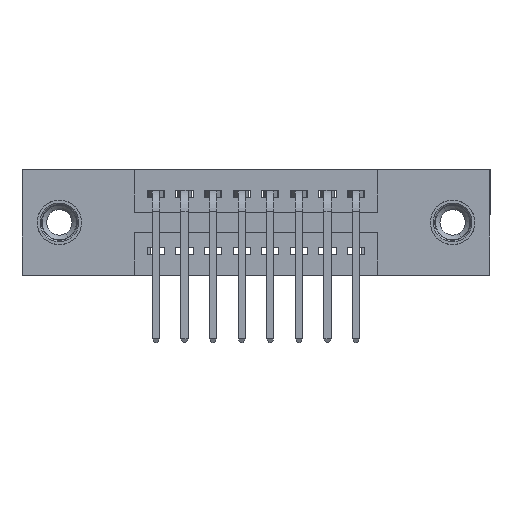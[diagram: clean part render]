
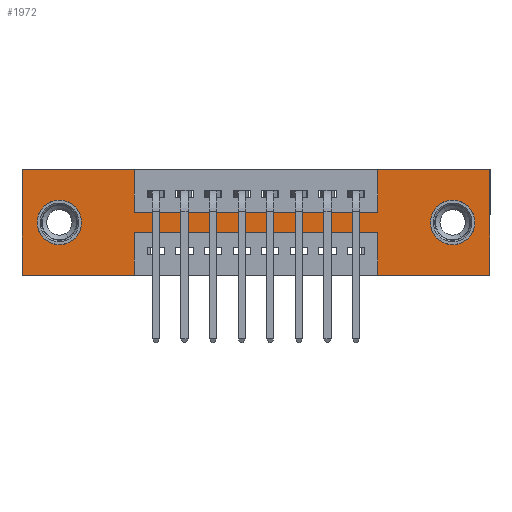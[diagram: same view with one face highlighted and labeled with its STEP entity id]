
A CAD part, front view. The second image highlights one B-rep face of the part: STEP entity #1972.
In plain terms, the highlighted planar face has unit normal (0, -1, 0).
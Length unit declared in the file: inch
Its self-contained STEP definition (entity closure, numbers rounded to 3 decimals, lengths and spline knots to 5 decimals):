
#18 = VECTOR ( 'NONE', #13733, 39.37008 ) ;
#299 = EDGE_LOOP ( 'NONE', ( #1664, #1999 ) ) ;
#496 = DIRECTION ( 'NONE',  ( 0., 1., 0. ) ) ;
#534 = DIRECTION ( 'NONE',  ( -1., 0., 0. ) ) ;
#543 = ORIENTED_EDGE ( 'NONE', *, *, #670, .F. ) ;
#641 = VECTOR ( 'NONE', #14571, 39.37008 ) ;
#670 = EDGE_CURVE ( 'NONE', #12947, #8249, #6791, .T. ) ;
#682 = EDGE_CURVE ( 'NONE', #10014, #4929, #6561, .T. ) ;
#694 = ORIENTED_EDGE ( 'NONE', *, *, #15339, .F. ) ;
#734 = CARTESIAN_POINT ( 'NONE',  ( 0., 0., 0. ) ) ;
#737 = CIRCLE ( 'NONE', #2516, 0.078 ) ;
#743 = LINE ( 'NONE', #13622, #641 ) ;
#760 = VECTOR ( 'NONE', #11612, 39.37008 ) ;
#789 = DIRECTION ( 'NONE',  ( 1., 0., 0. ) ) ;
#1268 = VERTEX_POINT ( 'NONE', #12419 ) ;
#1506 = LINE ( 'NONE', #7781, #1618 ) ;
#1618 = VECTOR ( 'NONE', #3947, 39.37008 ) ;
#1631 = EDGE_CURVE ( 'NONE', #8249, #10014, #2100, .T. ) ;
#1652 = FACE_OUTER_BOUND ( 'NONE', #6798, .T. ) ;
#1664 = ORIENTED_EDGE ( 'NONE', *, *, #5066, .T. ) ;
#1668 = FACE_BOUND ( 'NONE', #4876, .T. ) ;
#1741 = FACE_BOUND ( 'NONE', #299, .T. ) ;
#1745 = CARTESIAN_POINT ( 'NONE',  ( 1.2425, 0., -0.37 ) ) ;
#1769 = EDGE_CURVE ( 'NONE', #4929, #5615, #6262, .T. ) ;
#1861 = VECTOR ( 'NONE', #4377, 39.37008 ) ;
#1972 = ADVANCED_FACE ( 'NONE', ( #1741, #1668, #1652 ), #5849, .T. ) ;
#1999 = ORIENTED_EDGE ( 'NONE', *, *, #5285, .T. ) ;
#2100 = LINE ( 'NONE', #11479, #760 ) ;
#2164 = LINE ( 'NONE', #12662, #18 ) ;
#2399 = CARTESIAN_POINT ( 'NONE',  ( 0.3925, 0., -0.15 ) ) ;
#2436 = CARTESIAN_POINT ( 'NONE',  ( 1.635, 0., 0. ) ) ;
#2516 = AXIS2_PLACEMENT_3D ( 'NONE', #4756, #12965, #6006 ) ;
#2610 = CARTESIAN_POINT ( 'NONE',  ( 1.2425, 0., -0.37 ) ) ;
#3034 = CARTESIAN_POINT ( 'NONE',  ( 0.3925, 0., -0.15 ) ) ;
#3137 = CARTESIAN_POINT ( 'NONE',  ( 0.13, 0., -0.107 ) ) ;
#3434 = ORIENTED_EDGE ( 'NONE', *, *, #11686, .T. ) ;
#3501 = AXIS2_PLACEMENT_3D ( 'NONE', #7628, #15226, #8829 ) ;
#3505 = DIRECTION ( 'NONE',  ( 1., 0., 0. ) ) ;
#3509 = CARTESIAN_POINT ( 'NONE',  ( 0.3925, 0., -0.37 ) ) ;
#3586 = ORIENTED_EDGE ( 'NONE', *, *, #12918, .T. ) ;
#3690 = VERTEX_POINT ( 'NONE', #3509 ) ;
#3752 = ORIENTED_EDGE ( 'NONE', *, *, #8537, .F. ) ;
#3947 = DIRECTION ( 'NONE',  ( -1., 0., 0. ) ) ;
#3972 = ORIENTED_EDGE ( 'NONE', *, *, #8665, .F. ) ;
#4113 = DIRECTION ( 'NONE',  ( 0., 0., 1. ) ) ;
#4246 = CARTESIAN_POINT ( 'NONE',  ( 0., 0., 0. ) ) ;
#4321 = VECTOR ( 'NONE', #11413, 39.37008 ) ;
#4373 = DIRECTION ( 'NONE',  ( 1., 0., 0. ) ) ;
#4377 = DIRECTION ( 'NONE',  ( 0., 0., -1. ) ) ;
#4563 = CARTESIAN_POINT ( 'NONE',  ( 1.2425, 0., -0.15 ) ) ;
#4582 = VECTOR ( 'NONE', #8848, 39.37008 ) ;
#4652 = CARTESIAN_POINT ( 'NONE',  ( 0., 0., -0.37 ) ) ;
#4718 = LINE ( 'NONE', #9942, #4582 ) ;
#4756 = CARTESIAN_POINT ( 'NONE',  ( 1.505, 0., -0.185 ) ) ;
#4876 = EDGE_LOOP ( 'NONE', ( #3434, #3586 ) ) ;
#4929 = VERTEX_POINT ( 'NONE', #2436 ) ;
#5066 = EDGE_CURVE ( 'NONE', #1268, #8824, #737, .T. ) ;
#5101 = CIRCLE ( 'NONE', #13154, 0.078 ) ;
#5285 = EDGE_CURVE ( 'NONE', #8824, #1268, #5980, .T. ) ;
#5615 = VERTEX_POINT ( 'NONE', #11672 ) ;
#5686 = VERTEX_POINT ( 'NONE', #1745 ) ;
#5849 = PLANE ( 'NONE',  #14478 ) ;
#5980 = CIRCLE ( 'NONE', #8642, 0.078 ) ;
#6006 = DIRECTION ( 'NONE',  ( 0., 0., -1. ) ) ;
#6081 = CARTESIAN_POINT ( 'NONE',  ( 0.13, 0., -0.263 ) ) ;
#6229 = EDGE_CURVE ( 'NONE', #5686, #7236, #10957, .T. ) ;
#6262 = LINE ( 'NONE', #8775, #4321 ) ;
#6342 = EDGE_CURVE ( 'NONE', #6452, #7640, #2164, .T. ) ;
#6396 = CARTESIAN_POINT ( 'NONE',  ( 0.3925, 0., -0.22 ) ) ;
#6397 = VECTOR ( 'NONE', #4373, 39.37008 ) ;
#6452 = VERTEX_POINT ( 'NONE', #4652 ) ;
#6561 = LINE ( 'NONE', #4246, #6397 ) ;
#6646 = ORIENTED_EDGE ( 'NONE', *, *, #6342, .F. ) ;
#6791 = LINE ( 'NONE', #3034, #7049 ) ;
#6798 = EDGE_LOOP ( 'NONE', ( #3972, #8311, #9697, #12326, #14183, #14683, #14709, #543, #694, #3752, #6646, #7280 ) ) ;
#6810 = VECTOR ( 'NONE', #789, 39.37008 ) ;
#7049 = VECTOR ( 'NONE', #3505, 39.37008 ) ;
#7165 = LINE ( 'NONE', #734, #6810 ) ;
#7236 = VERTEX_POINT ( 'NONE', #13797 ) ;
#7280 = ORIENTED_EDGE ( 'NONE', *, *, #8046, .F. ) ;
#7583 = DIRECTION ( 'NONE',  ( 0., -1., 0. ) ) ;
#7628 = CARTESIAN_POINT ( 'NONE',  ( 0.13, 0., -0.185 ) ) ;
#7640 = VERTEX_POINT ( 'NONE', #14216 ) ;
#7781 = CARTESIAN_POINT ( 'NONE',  ( 0.3925, 0., -0.22 ) ) ;
#7786 = DIRECTION ( 'NONE',  ( 0., 1., 0. ) ) ;
#7861 = EDGE_CURVE ( 'NONE', #7236, #11448, #1506, .T. ) ;
#8046 = EDGE_CURVE ( 'NONE', #3690, #6452, #743, .T. ) ;
#8249 = VERTEX_POINT ( 'NONE', #4563 ) ;
#8311 = ORIENTED_EDGE ( 'NONE', *, *, #7861, .F. ) ;
#8475 = CARTESIAN_POINT ( 'NONE',  ( 0.13, 0., -0.185 ) ) ;
#8537 = EDGE_CURVE ( 'NONE', #7640, #9403, #7165, .T. ) ;
#8642 = AXIS2_PLACEMENT_3D ( 'NONE', #14421, #7786, #15325 ) ;
#8665 = EDGE_CURVE ( 'NONE', #11448, #3690, #4718, .T. ) ;
#8775 = CARTESIAN_POINT ( 'NONE',  ( 1.635, 0., 0. ) ) ;
#8824 = VERTEX_POINT ( 'NONE', #14167 ) ;
#8829 = DIRECTION ( 'NONE',  ( 0., 0., 1. ) ) ;
#8848 = DIRECTION ( 'NONE',  ( 0., 0., -1. ) ) ;
#9040 = CIRCLE ( 'NONE', #3501, 0.078 ) ;
#9333 = EDGE_CURVE ( 'NONE', #5615, #5686, #12052, .T. ) ;
#9403 = VERTEX_POINT ( 'NONE', #14148 ) ;
#9610 = DIRECTION ( 'NONE',  ( 0., 0., 1. ) ) ;
#9697 = ORIENTED_EDGE ( 'NONE', *, *, #6229, .F. ) ;
#9819 = CARTESIAN_POINT ( 'NONE',  ( 1.2425, 0., 0. ) ) ;
#9942 = CARTESIAN_POINT ( 'NONE',  ( 0.3925, 0., -0.37 ) ) ;
#9957 = VERTEX_POINT ( 'NONE', #6081 ) ;
#10014 = VERTEX_POINT ( 'NONE', #9819 ) ;
#10673 = VERTEX_POINT ( 'NONE', #3137 ) ;
#10792 = CARTESIAN_POINT ( 'NONE',  ( 0., 0., -0.37 ) ) ;
#10939 = VECTOR ( 'NONE', #4113, 39.37008 ) ;
#10957 = LINE ( 'NONE', #2610, #10939 ) ;
#11413 = DIRECTION ( 'NONE',  ( 0., 0., -1. ) ) ;
#11437 = CARTESIAN_POINT ( 'NONE',  ( 0., 0., -0.37 ) ) ;
#11448 = VERTEX_POINT ( 'NONE', #6396 ) ;
#11456 = LINE ( 'NONE', #13739, #1861 ) ;
#11479 = CARTESIAN_POINT ( 'NONE',  ( 1.2425, 0., 0. ) ) ;
#11612 = DIRECTION ( 'NONE',  ( 0., 0., 1. ) ) ;
#11672 = CARTESIAN_POINT ( 'NONE',  ( 1.635, 0., -0.37 ) ) ;
#11686 = EDGE_CURVE ( 'NONE', #10673, #9957, #5101, .T. ) ;
#11898 = VECTOR ( 'NONE', #534, 39.37008 ) ;
#12052 = LINE ( 'NONE', #10792, #11898 ) ;
#12204 = DIRECTION ( 'NONE',  ( 0., 0., -1. ) ) ;
#12326 = ORIENTED_EDGE ( 'NONE', *, *, #9333, .F. ) ;
#12419 = CARTESIAN_POINT ( 'NONE',  ( 1.505, 0., -0.107 ) ) ;
#12662 = CARTESIAN_POINT ( 'NONE',  ( 0., 0., 0. ) ) ;
#12918 = EDGE_CURVE ( 'NONE', #9957, #10673, #9040, .T. ) ;
#12947 = VERTEX_POINT ( 'NONE', #2399 ) ;
#12965 = DIRECTION ( 'NONE',  ( 0., 1., 0. ) ) ;
#13154 = AXIS2_PLACEMENT_3D ( 'NONE', #8475, #496, #9610 ) ;
#13622 = CARTESIAN_POINT ( 'NONE',  ( 0., 0., -0.37 ) ) ;
#13733 = DIRECTION ( 'NONE',  ( 0., 0., 1. ) ) ;
#13739 = CARTESIAN_POINT ( 'NONE',  ( 0.3925, 0., 0. ) ) ;
#13797 = CARTESIAN_POINT ( 'NONE',  ( 1.2425, 0., -0.22 ) ) ;
#14148 = CARTESIAN_POINT ( 'NONE',  ( 0.3925, 0., 0. ) ) ;
#14167 = CARTESIAN_POINT ( 'NONE',  ( 1.505, 0., -0.263 ) ) ;
#14183 = ORIENTED_EDGE ( 'NONE', *, *, #1769, .F. ) ;
#14216 = CARTESIAN_POINT ( 'NONE',  ( 0., 0., 0. ) ) ;
#14421 = CARTESIAN_POINT ( 'NONE',  ( 1.505, 0., -0.185 ) ) ;
#14478 = AXIS2_PLACEMENT_3D ( 'NONE', #11437, #7583, #12204 ) ;
#14571 = DIRECTION ( 'NONE',  ( -1., 0., 0. ) ) ;
#14683 = ORIENTED_EDGE ( 'NONE', *, *, #682, .F. ) ;
#14709 = ORIENTED_EDGE ( 'NONE', *, *, #1631, .F. ) ;
#15226 = DIRECTION ( 'NONE',  ( 0., 1., 0. ) ) ;
#15325 = DIRECTION ( 'NONE',  ( 0., 0., -1. ) ) ;
#15339 = EDGE_CURVE ( 'NONE', #9403, #12947, #11456, .T. ) ;
